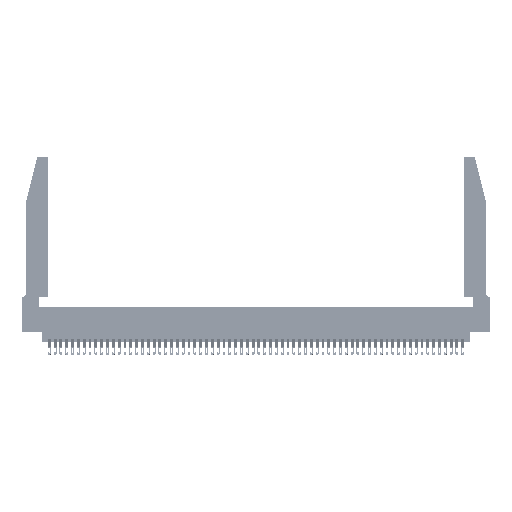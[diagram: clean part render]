
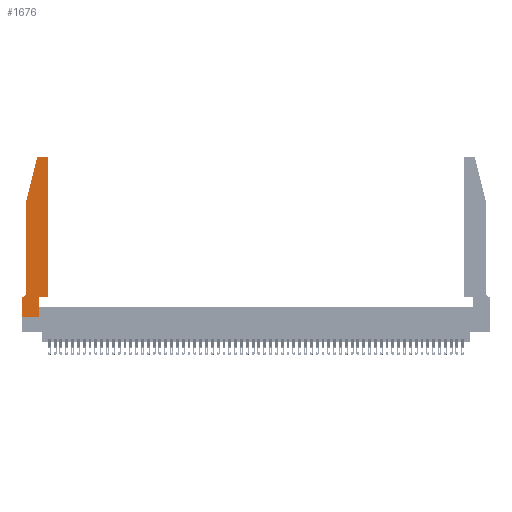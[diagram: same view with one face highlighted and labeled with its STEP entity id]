
A CAD part, top view. The second image highlights one B-rep face of the part: STEP entity #1676.
In plain terms, the highlighted planar face has unit normal (0, 0, 1).
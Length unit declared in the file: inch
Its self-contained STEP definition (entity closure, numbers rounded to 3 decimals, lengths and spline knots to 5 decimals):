
#67 = LINE ( 'NONE', #35250, #47560 ) ;
#240 = VERTEX_POINT ( 'NONE', #41165 ) ;
#268 = CIRCLE ( 'NONE', #34634, 0.07 ) ;
#1676 = ADVANCED_FACE ( 'NONE', ( #41160 ), #41807, .T. ) ;
#1714 = ORIENTED_EDGE ( 'NONE', *, *, #11658, .T. ) ;
#1966 = CARTESIAN_POINT ( 'NONE',  ( 0., 0., 0.37 ) ) ;
#2147 = CARTESIAN_POINT ( 'NONE',  ( 0.4505, 0.35, 0.37 ) ) ;
#2407 = LINE ( 'NONE', #5715, #36639 ) ;
#3048 = EDGE_CURVE ( 'NONE', #19341, #13807, #67, .T. ) ;
#4302 = VECTOR ( 'NONE', #55359, 39.37008 ) ;
#5633 = CARTESIAN_POINT ( 'NONE',  ( 0.284, 2.72, 0.37 ) ) ;
#5696 = LINE ( 'NONE', #1966, #4302 ) ;
#5715 = CARTESIAN_POINT ( 'NONE',  ( 0.0755, 0.35, 0.37 ) ) ;
#5858 = CARTESIAN_POINT ( 'NONE',  ( 0.0055, 0.42, 0.37 ) ) ;
#6218 = ORIENTED_EDGE ( 'NONE', *, *, #36489, .T. ) ;
#6990 = EDGE_CURVE ( 'NONE', #37917, #33470, #29812, .T. ) ;
#7178 = ORIENTED_EDGE ( 'NONE', *, *, #24848, .T. ) ;
#7524 = AXIS2_PLACEMENT_3D ( 'NONE', #15171, #19660, #50719 ) ;
#7633 = EDGE_CURVE ( 'NONE', #13807, #16732, #268, .T. ) ;
#8074 = ORIENTED_EDGE ( 'NONE', *, *, #7633, .T. ) ;
#8163 = VERTEX_POINT ( 'NONE', #9161 ) ;
#8805 = VECTOR ( 'NONE', #29997, 39.37008 ) ;
#8979 = VERTEX_POINT ( 'NONE', #21694 ) ;
#9161 = CARTESIAN_POINT ( 'NONE',  ( 0.25487, 2.72718, 0.37 ) ) ;
#9885 = DIRECTION ( 'NONE',  ( -1., 0., 0. ) ) ;
#10182 = DIRECTION ( 'NONE',  ( 1., 0., 0. ) ) ;
#10224 = LINE ( 'NONE', #16547, #8805 ) ;
#10273 = DIRECTION ( 'NONE',  ( -1., 0., 0. ) ) ;
#10415 = DIRECTION ( 'NONE',  ( -1., 0., 0. ) ) ;
#10913 = AXIS2_PLACEMENT_3D ( 'NONE', #5633, #36854, #10182 ) ;
#11255 = EDGE_CURVE ( 'NONE', #8163, #19341, #10224, .T. ) ;
#11658 = EDGE_CURVE ( 'NONE', #16732, #52858, #2407, .T. ) ;
#12202 = ORIENTED_EDGE ( 'NONE', *, *, #3048, .T. ) ;
#12663 = LINE ( 'NONE', #32405, #34963 ) ;
#12722 = VECTOR ( 'NONE', #38858, 39.37008 ) ;
#13365 = EDGE_CURVE ( 'NONE', #42586, #37917, #46179, .T. ) ;
#13807 = VERTEX_POINT ( 'NONE', #37909 ) ;
#13989 = ORIENTED_EDGE ( 'NONE', *, *, #11255, .T. ) ;
#14383 = CARTESIAN_POINT ( 'NONE',  ( 0.2605, 2.75, 0.37 ) ) ;
#14788 = CARTESIAN_POINT ( 'NONE',  ( 0.2865, 0., 0.37 ) ) ;
#15171 = CARTESIAN_POINT ( 'NONE',  ( 0., 0.35, 0.37 ) ) ;
#15197 = EDGE_CURVE ( 'NONE', #37291, #8979, #48197, .T. ) ;
#16547 = CARTESIAN_POINT ( 'NONE',  ( 0.0755, 2., 0.37 ) ) ;
#16732 = VERTEX_POINT ( 'NONE', #23363 ) ;
#19341 = VERTEX_POINT ( 'NONE', #36764 ) ;
#19522 = ORIENTED_EDGE ( 'NONE', *, *, #38781, .T. ) ;
#19660 = DIRECTION ( 'NONE',  ( 0., 0., 1. ) ) ;
#20556 = ORIENTED_EDGE ( 'NONE', *, *, #13365, .T. ) ;
#21694 = CARTESIAN_POINT ( 'NONE',  ( 0.2865, 0.35, 0.37 ) ) ;
#23363 = CARTESIAN_POINT ( 'NONE',  ( 0.0055, 0.35, 0.37 ) ) ;
#24848 = EDGE_CURVE ( 'NONE', #240, #42586, #25827, .T. ) ;
#25827 = LINE ( 'NONE', #2147, #36224 ) ;
#26126 = DIRECTION ( 'NONE',  ( 0., 0., 1. ) ) ;
#26635 = AXIS2_PLACEMENT_3D ( 'NONE', #52693, #26126, #57117 ) ;
#29812 = LINE ( 'NONE', #14383, #52032 ) ;
#29997 = DIRECTION ( 'NONE',  ( -0.239, -0.971, 0. ) ) ;
#31196 = LINE ( 'NONE', #47691, #33968 ) ;
#32405 = CARTESIAN_POINT ( 'NONE',  ( 0.4505, 0.35, 0.37 ) ) ;
#33470 = VERTEX_POINT ( 'NONE', #34846 ) ;
#33968 = VECTOR ( 'NONE', #52149, 39.37008 ) ;
#34399 = CARTESIAN_POINT ( 'NONE',  ( 0.2865, 0.35, 0.37 ) ) ;
#34634 = AXIS2_PLACEMENT_3D ( 'NONE', #5858, #37064, #10415 ) ;
#34846 = CARTESIAN_POINT ( 'NONE',  ( 0.284, 2.75, 0.37 ) ) ;
#34963 = VECTOR ( 'NONE', #36840, 39.37008 ) ;
#35250 = CARTESIAN_POINT ( 'NONE',  ( 0.0755, 2., 0.37 ) ) ;
#36224 = VECTOR ( 'NONE', #37893, 39.37008 ) ;
#36489 = EDGE_CURVE ( 'NONE', #8979, #240, #12663, .T. ) ;
#36639 = VECTOR ( 'NONE', #10273, 39.37008 ) ;
#36764 = CARTESIAN_POINT ( 'NONE',  ( 0.0755, 2., 0.37 ) ) ;
#36840 = DIRECTION ( 'NONE',  ( 1., 0., 0. ) ) ;
#36854 = DIRECTION ( 'NONE',  ( 0., 0., 1. ) ) ;
#37064 = DIRECTION ( 'NONE',  ( 0., 0., -1. ) ) ;
#37291 = VERTEX_POINT ( 'NONE', #14788 ) ;
#37893 = DIRECTION ( 'NONE',  ( 0., 1., 0. ) ) ;
#37909 = CARTESIAN_POINT ( 'NONE',  ( 0.0755, 0.42, 0.37 ) ) ;
#37917 = VERTEX_POINT ( 'NONE', #46235 ) ;
#38195 = ORIENTED_EDGE ( 'NONE', *, *, #55191, .T. ) ;
#38414 = CARTESIAN_POINT ( 'NONE',  ( 0., 0., 0.37 ) ) ;
#38781 = EDGE_CURVE ( 'NONE', #55950, #37291, #31196, .T. ) ;
#38858 = DIRECTION ( 'NONE',  ( 0., 1., 0. ) ) ;
#41160 = FACE_OUTER_BOUND ( 'NONE', #44685, .T. ) ;
#41165 = CARTESIAN_POINT ( 'NONE',  ( 0.4505, 0.35, 0.37 ) ) ;
#41807 = PLANE ( 'NONE',  #7524 ) ;
#42586 = VERTEX_POINT ( 'NONE', #52402 ) ;
#44654 = EDGE_CURVE ( 'NONE', #33470, #8163, #51736, .T. ) ;
#44685 = EDGE_LOOP ( 'NONE', ( #46045, #48079, #13989, #12202, #8074, #1714, #38195, #19522, #52212, #6218, #7178, #20556 ) ) ;
#45461 = CARTESIAN_POINT ( 'NONE',  ( 0., 0.35, 0.37 ) ) ;
#46045 = ORIENTED_EDGE ( 'NONE', *, *, #6990, .T. ) ;
#46179 = CIRCLE ( 'NONE', #26635, 0.03 ) ;
#46235 = CARTESIAN_POINT ( 'NONE',  ( 0.4205, 2.75, 0.37 ) ) ;
#47560 = VECTOR ( 'NONE', #48616, 39.37008 ) ;
#47691 = CARTESIAN_POINT ( 'NONE',  ( 0., 0., 0.37 ) ) ;
#48079 = ORIENTED_EDGE ( 'NONE', *, *, #44654, .T. ) ;
#48197 = LINE ( 'NONE', #34399, #12722 ) ;
#48616 = DIRECTION ( 'NONE',  ( 0., -1., 0. ) ) ;
#50719 = DIRECTION ( 'NONE',  ( 1., 0., 0. ) ) ;
#51736 = CIRCLE ( 'NONE', #10913, 0.03 ) ;
#52032 = VECTOR ( 'NONE', #9885, 39.37008 ) ;
#52149 = DIRECTION ( 'NONE',  ( 1., 0., 0. ) ) ;
#52212 = ORIENTED_EDGE ( 'NONE', *, *, #15197, .T. ) ;
#52402 = CARTESIAN_POINT ( 'NONE',  ( 0.4505, 2.72, 0.37 ) ) ;
#52693 = CARTESIAN_POINT ( 'NONE',  ( 0.4205, 2.72, 0.37 ) ) ;
#52858 = VERTEX_POINT ( 'NONE', #45461 ) ;
#55191 = EDGE_CURVE ( 'NONE', #52858, #55950, #5696, .T. ) ;
#55359 = DIRECTION ( 'NONE',  ( 0., -1., 0. ) ) ;
#55950 = VERTEX_POINT ( 'NONE', #38414 ) ;
#57117 = DIRECTION ( 'NONE',  ( 1., 0., 0. ) ) ;
